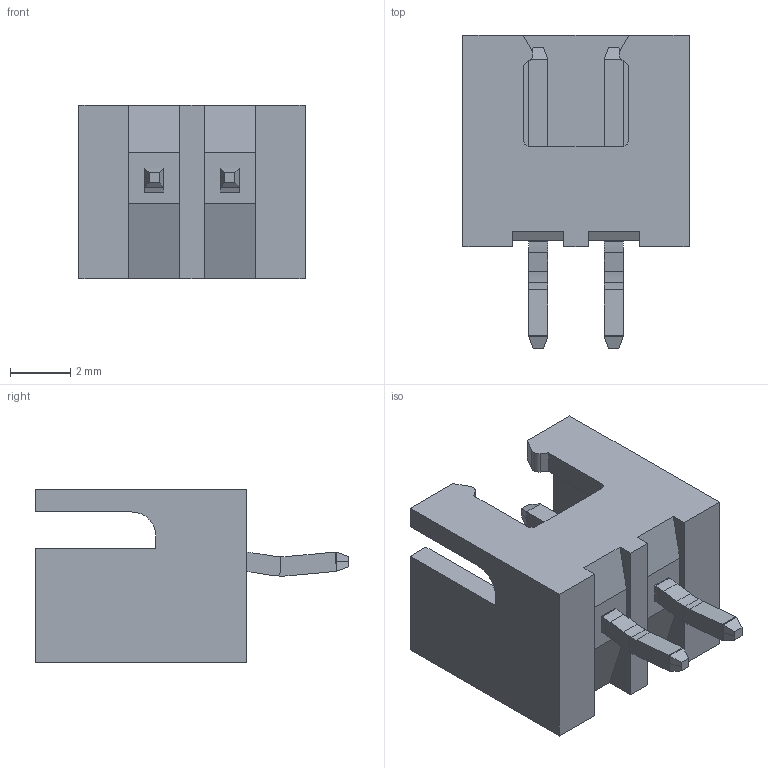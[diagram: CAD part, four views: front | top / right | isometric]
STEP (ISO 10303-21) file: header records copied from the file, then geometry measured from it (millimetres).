
FILE_DESCRIPTION (( 'STEP AP203' ), '1' );
FILE_NAME ('14K-502-412-AA1.STEP', '2024-02-23T17:06:00', ( '' ), ( '' ), 'SwSTEP 2.0', 'SolidWorks 2023', '' );
FILE_SCHEMA (( 'CONFIG_CONTROL_DESIGN' ));
Length unit declared in the file: millimetre
Products named in the file (3): 14K Series Pin_12; 14K Series Pin Header Insulator_502; 14K-502-412-AA1
Assembly tree (3 placements, depth 2):
  14K-502-412-AA1
    14K Series Pin Header Insulator_502
    14K Series Pin_12  x2
Bounding box: 7.5 x 10.4 x 5.75 mm (x, y, z)
Volume: 152 mm3; surface area: 415.4 mm2
Topology: 3 solids, 3 shells, 122 faces, 324 edges, 208 vertices
Faces by surface type: plane 103, cylinder 19
Entity records: 3087 total; most frequent: CARTESIAN_POINT 490, ORIENTED_EDGE 480, DIRECTION 462, EDGE_CURVE 240, LINE 206, VECTOR 206, VERTEX_POINT 156, AXIS2_PLACEMENT_3D 128
